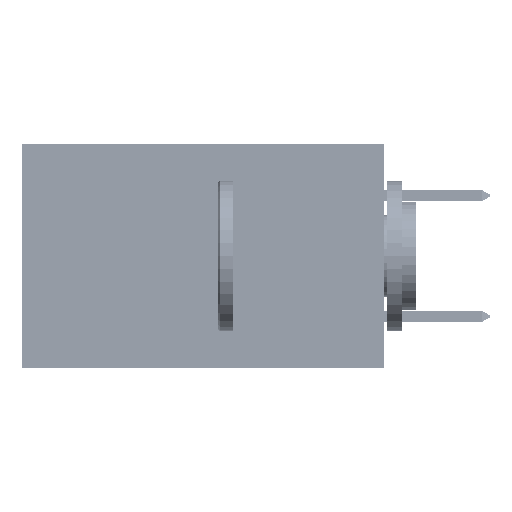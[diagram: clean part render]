
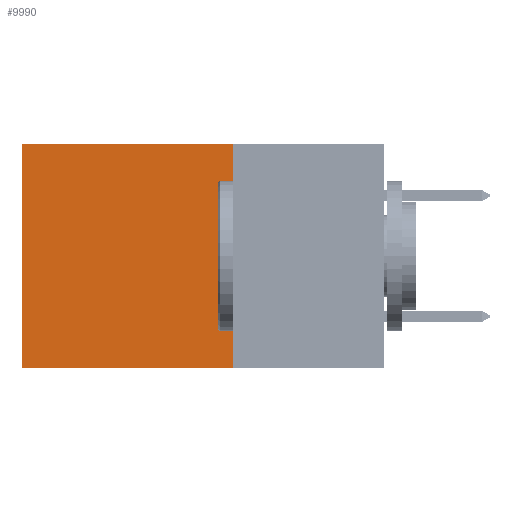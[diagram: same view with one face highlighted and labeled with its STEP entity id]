
A CAD part, left-side view. The second image highlights one B-rep face of the part: STEP entity #9990.
In plain terms, the highlighted planar face has unit normal (-1, 0, 0).
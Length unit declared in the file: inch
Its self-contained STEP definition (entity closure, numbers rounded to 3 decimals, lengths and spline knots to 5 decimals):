
#50 = EDGE_CURVE ( 'NONE', #43371, #36998, #11937, .T. ) ;
#577 = CARTESIAN_POINT ( 'NONE',  ( 0.2875, 0.6, -0.37 ) ) ;
#1242 = VERTEX_POINT ( 'NONE', #38183 ) ;
#2791 = DIRECTION ( 'NONE',  ( 0., 1., 0. ) ) ;
#3777 = DIRECTION ( 'NONE',  ( 0., 1., 0. ) ) ;
#4201 = VERTEX_POINT ( 'NONE', #577 ) ;
#4414 = DIRECTION ( 'NONE',  ( 1., 0., 0. ) ) ;
#4639 = VECTOR ( 'NONE', #3777, 39.37008 ) ;
#5221 = EDGE_CURVE ( 'NONE', #43371, #1242, #5398, .T. ) ;
#5398 = LINE ( 'NONE', #44383, #40559 ) ;
#7265 = CARTESIAN_POINT ( 'NONE',  ( 0.2875, 0.25, -0.37 ) ) ;
#9990 = ADVANCED_FACE ( 'NONE', ( #12855 ), #14759, .F. ) ;
#10144 = LINE ( 'NONE', #39005, #37118 ) ;
#10427 = EDGE_CURVE ( 'NONE', #1242, #4201, #32648, .T. ) ;
#11937 = LINE ( 'NONE', #34364, #29559 ) ;
#12855 = FACE_OUTER_BOUND ( 'NONE', #23495, .T. ) ;
#14369 = DIRECTION ( 'NONE',  ( 0., 0., -1. ) ) ;
#14759 = PLANE ( 'NONE',  #44121 ) ;
#15399 = ORIENTED_EDGE ( 'NONE', *, *, #5221, .F. ) ;
#22292 = ORIENTED_EDGE ( 'NONE', *, *, #50, .T. ) ;
#23495 = EDGE_LOOP ( 'NONE', ( #39835, #24596, #15399, #22292 ) ) ;
#24596 = ORIENTED_EDGE ( 'NONE', *, *, #10427, .F. ) ;
#25185 = EDGE_CURVE ( 'NONE', #36998, #4201, #10144, .T. ) ;
#26719 = DIRECTION ( 'NONE',  ( 0., 0., -1. ) ) ;
#28942 = DIRECTION ( 'NONE',  ( 0., 0., -1. ) ) ;
#29559 = VECTOR ( 'NONE', #2791, 39.37008 ) ;
#32648 = LINE ( 'NONE', #7265, #4639 ) ;
#34364 = CARTESIAN_POINT ( 'NONE',  ( 0.2875, 0.25, 0. ) ) ;
#36998 = VERTEX_POINT ( 'NONE', #40776 ) ;
#37118 = VECTOR ( 'NONE', #14369, 39.37008 ) ;
#38183 = CARTESIAN_POINT ( 'NONE',  ( 0.2875, 0.25, -0.37 ) ) ;
#38268 = CARTESIAN_POINT ( 'NONE',  ( 0.2875, 0.25, 0. ) ) ;
#39005 = CARTESIAN_POINT ( 'NONE',  ( 0.2875, 0.6, 0. ) ) ;
#39403 = CARTESIAN_POINT ( 'NONE',  ( 0.2875, 0.25, 0. ) ) ;
#39835 = ORIENTED_EDGE ( 'NONE', *, *, #25185, .T. ) ;
#40559 = VECTOR ( 'NONE', #26719, 39.37008 ) ;
#40776 = CARTESIAN_POINT ( 'NONE',  ( 0.2875, 0.6, 0. ) ) ;
#43371 = VERTEX_POINT ( 'NONE', #38268 ) ;
#44121 = AXIS2_PLACEMENT_3D ( 'NONE', #39403, #4414, #28942 ) ;
#44383 = CARTESIAN_POINT ( 'NONE',  ( 0.2875, 0.25, 0. ) ) ;
